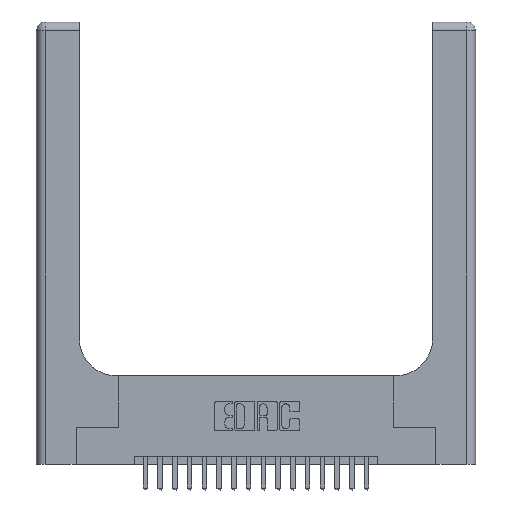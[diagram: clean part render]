
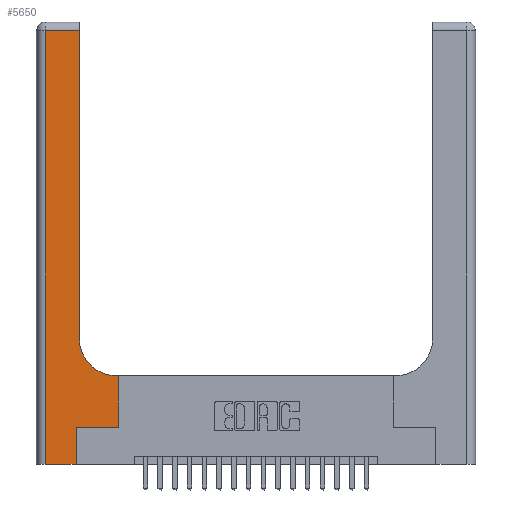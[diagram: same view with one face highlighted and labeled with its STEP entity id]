
A CAD part, top view. The second image highlights one B-rep face of the part: STEP entity #5650.
In plain terms, the highlighted planar face has unit normal (0, 0, 1).
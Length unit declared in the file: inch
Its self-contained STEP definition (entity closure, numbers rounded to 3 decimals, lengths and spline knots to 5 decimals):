
#502 = VERTEX_POINT ( 'NONE', #7329 ) ;
#1239 = DIRECTION ( 'NONE',  ( 0., 1., 0. ) ) ;
#2318 = CARTESIAN_POINT ( 'NONE',  ( 0., 0., 0.37 ) ) ;
#2489 = VECTOR ( 'NONE', #1239, 39.37008 ) ;
#2785 = AXIS2_PLACEMENT_3D ( 'NONE', #17686, #20872, #11112 ) ;
#3670 = CARTESIAN_POINT ( 'NONE',  ( 0., 2.94, 0.37 ) ) ;
#3706 = VERTEX_POINT ( 'NONE', #18512 ) ;
#3826 = EDGE_LOOP ( 'NONE', ( #15168, #18428, #16423, #15514, #19628, #11932, #20401, #12027, #19457 ) ) ;
#4079 = LINE ( 'NONE', #2318, #11797 ) ;
#4485 = DIRECTION ( 'NONE',  ( 1., 0., 0. ) ) ;
#4935 = FACE_OUTER_BOUND ( 'NONE', #3826, .T. ) ;
#4987 = VERTEX_POINT ( 'NONE', #7656 ) ;
#5131 = DIRECTION ( 'NONE',  ( 0., 0., -1. ) ) ;
#5535 = VERTEX_POINT ( 'NONE', #20533 ) ;
#5539 = VERTEX_POINT ( 'NONE', #19021 ) ;
#5650 = ADVANCED_FACE ( 'NONE', ( #4935 ), #19295, .F. ) ;
#5888 = EDGE_CURVE ( 'NONE', #7605, #4987, #18290, .T. ) ;
#6113 = VECTOR ( 'NONE', #13540, 39.37008 ) ;
#6178 = VERTEX_POINT ( 'NONE', #8797 ) ;
#6276 = VERTEX_POINT ( 'NONE', #7482 ) ;
#6436 = EDGE_CURVE ( 'NONE', #5539, #6178, #13908, .T. ) ;
#7329 = CARTESIAN_POINT ( 'NONE',  ( 0.06, 0., 0.37 ) ) ;
#7482 = CARTESIAN_POINT ( 'NONE',  ( 0.269, 0., 0.37 ) ) ;
#7605 = VERTEX_POINT ( 'NONE', #11271 ) ;
#7628 = CARTESIAN_POINT ( 'NONE',  ( 0.2915, 3., 0.37 ) ) ;
#7656 = CARTESIAN_POINT ( 'NONE',  ( 0.2915, 0.85, 0.37 ) ) ;
#8016 = EDGE_CURVE ( 'NONE', #4987, #5535, #14393, .T. ) ;
#8797 = CARTESIAN_POINT ( 'NONE',  ( 0.5585, 0.25, 0.37 ) ) ;
#9007 = EDGE_CURVE ( 'NONE', #3706, #502, #20935, .T. ) ;
#9826 = VERTEX_POINT ( 'NONE', #14366 ) ;
#10270 = DIRECTION ( 'NONE',  ( 0., -1., 0. ) ) ;
#10286 = LINE ( 'NONE', #16495, #14692 ) ;
#11112 = DIRECTION ( 'NONE',  ( -1., 0., 0. ) ) ;
#11165 = EDGE_CURVE ( 'NONE', #9826, #7605, #10286, .T. ) ;
#11205 = CARTESIAN_POINT ( 'NONE',  ( 0.269, 0., 0.37 ) ) ;
#11271 = CARTESIAN_POINT ( 'NONE',  ( 0.5415, 0.6, 0.37 ) ) ;
#11797 = VECTOR ( 'NONE', #13890, 39.37008 ) ;
#11932 = ORIENTED_EDGE ( 'NONE', *, *, #6436, .T. ) ;
#12027 = ORIENTED_EDGE ( 'NONE', *, *, #11165, .T. ) ;
#12549 = EDGE_CURVE ( 'NONE', #502, #6276, #4079, .T. ) ;
#12841 = VECTOR ( 'NONE', #16889, 39.37008 ) ;
#13165 = DIRECTION ( 'NONE',  ( -1., 0., 0. ) ) ;
#13197 = EDGE_CURVE ( 'NONE', #6276, #5539, #20486, .T. ) ;
#13540 = DIRECTION ( 'NONE',  ( -1., 0., 0. ) ) ;
#13541 = EDGE_CURVE ( 'NONE', #6178, #9826, #17222, .T. ) ;
#13890 = DIRECTION ( 'NONE',  ( 1., 0., 0. ) ) ;
#13908 = LINE ( 'NONE', #16011, #17276 ) ;
#14366 = CARTESIAN_POINT ( 'NONE',  ( 0.5585, 0.6, 0.37 ) ) ;
#14393 = LINE ( 'NONE', #7628, #18238 ) ;
#14692 = VECTOR ( 'NONE', #13165, 39.37008 ) ;
#14981 = CARTESIAN_POINT ( 'NONE',  ( 0.5415, 0.85, 0.37 ) ) ;
#15168 = ORIENTED_EDGE ( 'NONE', *, *, #8016, .T. ) ;
#15185 = CARTESIAN_POINT ( 'NONE',  ( 0.06, 3., 0.37 ) ) ;
#15212 = CARTESIAN_POINT ( 'NONE',  ( 0.5585, 0.25, 0.37 ) ) ;
#15344 = LINE ( 'NONE', #3670, #6113 ) ;
#15514 = ORIENTED_EDGE ( 'NONE', *, *, #12549, .T. ) ;
#16011 = CARTESIAN_POINT ( 'NONE',  ( 0.269, 0.25, 0.37 ) ) ;
#16423 = ORIENTED_EDGE ( 'NONE', *, *, #9007, .T. ) ;
#16495 = CARTESIAN_POINT ( 'NONE',  ( 0.2915, 0.6, 0.37 ) ) ;
#16658 = DIRECTION ( 'NONE',  ( 1., 0., 0. ) ) ;
#16675 = VECTOR ( 'NONE', #10270, 39.37008 ) ;
#16889 = DIRECTION ( 'NONE',  ( 0., 1., 0. ) ) ;
#17222 = LINE ( 'NONE', #15212, #12841 ) ;
#17276 = VECTOR ( 'NONE', #4485, 39.37008 ) ;
#17686 = CARTESIAN_POINT ( 'NONE',  ( 0., 3., 0.37 ) ) ;
#18238 = VECTOR ( 'NONE', #19087, 39.37008 ) ;
#18263 = AXIS2_PLACEMENT_3D ( 'NONE', #14981, #5131, #16658 ) ;
#18290 = CIRCLE ( 'NONE', #18263, 0.25 ) ;
#18428 = ORIENTED_EDGE ( 'NONE', *, *, #18774, .T. ) ;
#18512 = CARTESIAN_POINT ( 'NONE',  ( 0.06, 2.94, 0.37 ) ) ;
#18774 = EDGE_CURVE ( 'NONE', #5535, #3706, #15344, .T. ) ;
#19021 = CARTESIAN_POINT ( 'NONE',  ( 0.269, 0.25, 0.37 ) ) ;
#19087 = DIRECTION ( 'NONE',  ( 0., 1., 0. ) ) ;
#19295 = PLANE ( 'NONE',  #2785 ) ;
#19457 = ORIENTED_EDGE ( 'NONE', *, *, #5888, .T. ) ;
#19628 = ORIENTED_EDGE ( 'NONE', *, *, #13197, .T. ) ;
#20401 = ORIENTED_EDGE ( 'NONE', *, *, #13541, .T. ) ;
#20486 = LINE ( 'NONE', #11205, #2489 ) ;
#20533 = CARTESIAN_POINT ( 'NONE',  ( 0.2915, 2.94, 0.37 ) ) ;
#20872 = DIRECTION ( 'NONE',  ( 0., 0., -1. ) ) ;
#20935 = LINE ( 'NONE', #15185, #16675 ) ;
